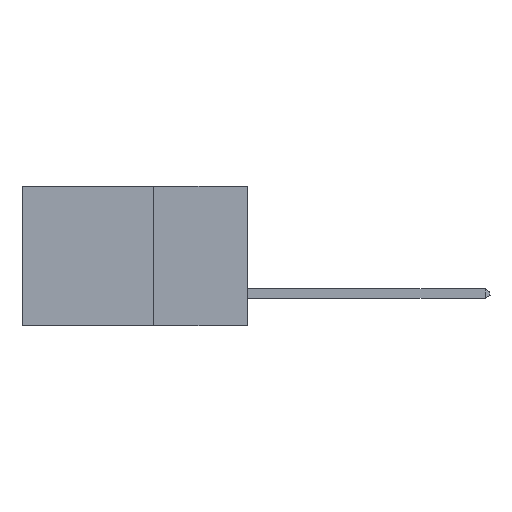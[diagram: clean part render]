
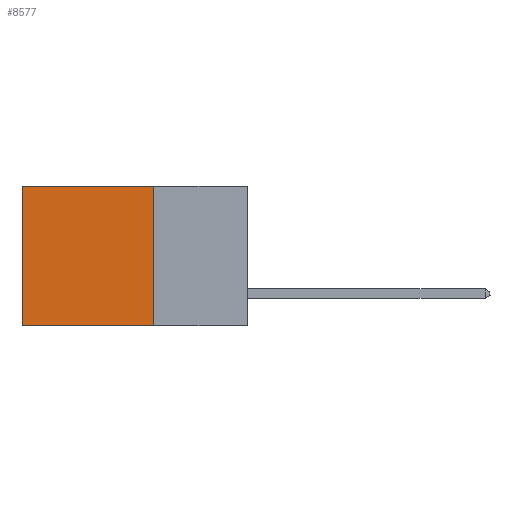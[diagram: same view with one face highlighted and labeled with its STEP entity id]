
A CAD part, left-side view. The second image highlights one B-rep face of the part: STEP entity #8577.
In plain terms, the highlighted planar face has unit normal (-1, 0, 0).
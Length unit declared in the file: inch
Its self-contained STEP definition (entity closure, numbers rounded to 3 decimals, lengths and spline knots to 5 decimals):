
#119 = ORIENTED_EDGE ( 'NONE', *, *, #14194, .F. ) ;
#179 = CARTESIAN_POINT ( 'NONE',  ( 0.298, 0.6, -0.37 ) ) ;
#195 = EDGE_CURVE ( 'NONE', #13220, #2803, #12910, .T. ) ;
#1297 = CARTESIAN_POINT ( 'NONE',  ( 0.298, 0.25, 0. ) ) ;
#1469 = VERTEX_POINT ( 'NONE', #8818 ) ;
#1578 = DIRECTION ( 'NONE',  ( 0., 1., 0. ) ) ;
#1768 = VECTOR ( 'NONE', #1578, 39.37008 ) ;
#1869 = EDGE_CURVE ( 'NONE', #7571, #13220, #2677, .T. ) ;
#2133 = ORIENTED_EDGE ( 'NONE', *, *, #195, .T. ) ;
#2677 = LINE ( 'NONE', #1297, #5887 ) ;
#2803 = VERTEX_POINT ( 'NONE', #179 ) ;
#2971 = VECTOR ( 'NONE', #15097, 39.37008 ) ;
#3468 = AXIS2_PLACEMENT_3D ( 'NONE', #13049, #8458, #14344 ) ;
#5505 = ORIENTED_EDGE ( 'NONE', *, *, #1869, .T. ) ;
#5887 = VECTOR ( 'NONE', #11400, 39.37008 ) ;
#5931 = DIRECTION ( 'NONE',  ( 0., 0., -1. ) ) ;
#6643 = CARTESIAN_POINT ( 'NONE',  ( 0.298, 0.6, 0. ) ) ;
#7317 = CARTESIAN_POINT ( 'NONE',  ( 0.298, 0.6, 0. ) ) ;
#7571 = VERTEX_POINT ( 'NONE', #13155 ) ;
#8458 = DIRECTION ( 'NONE',  ( 1., 0., 0. ) ) ;
#8577 = ADVANCED_FACE ( 'NONE', ( #12563 ), #11807, .F. ) ;
#8818 = CARTESIAN_POINT ( 'NONE',  ( 0.298, 0.25, -0.37 ) ) ;
#9564 = LINE ( 'NONE', #15722, #1768 ) ;
#9900 = ORIENTED_EDGE ( 'NONE', *, *, #12324, .F. ) ;
#10101 = CARTESIAN_POINT ( 'NONE',  ( 0.298, 0.25, 0. ) ) ;
#10760 = LINE ( 'NONE', #10101, #2971 ) ;
#10827 = EDGE_LOOP ( 'NONE', ( #2133, #9900, #119, #5505 ) ) ;
#11400 = DIRECTION ( 'NONE',  ( 0., 1., 0. ) ) ;
#11807 = PLANE ( 'NONE',  #3468 ) ;
#12324 = EDGE_CURVE ( 'NONE', #1469, #2803, #9564, .T. ) ;
#12563 = FACE_OUTER_BOUND ( 'NONE', #10827, .T. ) ;
#12910 = LINE ( 'NONE', #7317, #15886 ) ;
#13049 = CARTESIAN_POINT ( 'NONE',  ( 0.298, 0.25, 0. ) ) ;
#13155 = CARTESIAN_POINT ( 'NONE',  ( 0.298, 0.25, 0. ) ) ;
#13220 = VERTEX_POINT ( 'NONE', #6643 ) ;
#14194 = EDGE_CURVE ( 'NONE', #7571, #1469, #10760, .T. ) ;
#14344 = DIRECTION ( 'NONE',  ( 0., 0., -1. ) ) ;
#15097 = DIRECTION ( 'NONE',  ( 0., 0., -1. ) ) ;
#15722 = CARTESIAN_POINT ( 'NONE',  ( 0.298, 0.25, -0.37 ) ) ;
#15886 = VECTOR ( 'NONE', #5931, 39.37008 ) ;
